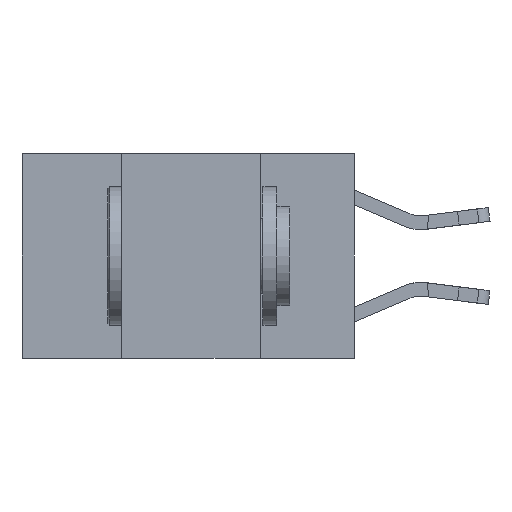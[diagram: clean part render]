
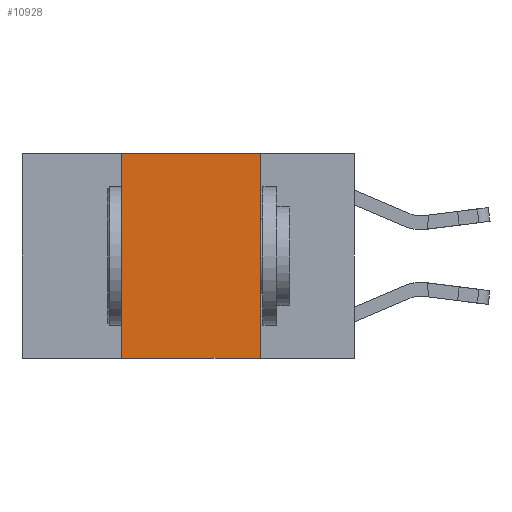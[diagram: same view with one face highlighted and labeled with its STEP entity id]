
A CAD part, left-side view. The second image highlights one B-rep face of the part: STEP entity #10928.
In plain terms, the highlighted planar face has unit normal (-1, 0, 0).
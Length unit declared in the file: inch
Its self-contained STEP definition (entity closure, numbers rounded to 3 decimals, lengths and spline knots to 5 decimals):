
#56 = VERTEX_POINT ( 'NONE', #12856 ) ;
#953 = CARTESIAN_POINT ( 'NONE',  ( 0., 0.6, -0.37 ) ) ;
#1276 = PLANE ( 'NONE',  #14299 ) ;
#2473 = DIRECTION ( 'NONE',  ( 0., -1., 0. ) ) ;
#2600 = DIRECTION ( 'NONE',  ( 1., 0., 0. ) ) ;
#2632 = ORIENTED_EDGE ( 'NONE', *, *, #9256, .F. ) ;
#3325 = LINE ( 'NONE', #12449, #12921 ) ;
#3659 = CARTESIAN_POINT ( 'NONE',  ( 0., 0.42, 0. ) ) ;
#4033 = ORIENTED_EDGE ( 'NONE', *, *, #9670, .F. ) ;
#4121 = ORIENTED_EDGE ( 'NONE', *, *, #9251, .F. ) ;
#5117 = ORIENTED_EDGE ( 'NONE', *, *, #9229, .T. ) ;
#6235 = DIRECTION ( 'NONE',  ( 0., -1., 0. ) ) ;
#6783 = VECTOR ( 'NONE', #6235, 39.37008 ) ;
#7540 = DIRECTION ( 'NONE',  ( 0., 0., -1. ) ) ;
#7731 = CARTESIAN_POINT ( 'NONE',  ( 0., 0.6, 0. ) ) ;
#7838 = VERTEX_POINT ( 'NONE', #14112 ) ;
#9226 = CARTESIAN_POINT ( 'NONE',  ( 0., 0.17, -0.37 ) ) ;
#9229 = EDGE_CURVE ( 'NONE', #7838, #14200, #10879, .T. ) ;
#9251 = EDGE_CURVE ( 'NONE', #7838, #10206, #10136, .T. ) ;
#9256 = EDGE_CURVE ( 'NONE', #56, #14200, #3325, .T. ) ;
#9670 = EDGE_CURVE ( 'NONE', #10206, #56, #14014, .T. ) ;
#9770 = VECTOR ( 'NONE', #13605, 39.37008 ) ;
#10136 = LINE ( 'NONE', #3659, #9770 ) ;
#10206 = VERTEX_POINT ( 'NONE', #11046 ) ;
#10664 = EDGE_LOOP ( 'NONE', ( #2632, #4033, #4121, #5117 ) ) ;
#10879 = LINE ( 'NONE', #953, #6783 ) ;
#10882 = VECTOR ( 'NONE', #2473, 39.37008 ) ;
#10928 = ADVANCED_FACE ( 'NONE', ( #15238 ), #1276, .F. ) ;
#11046 = CARTESIAN_POINT ( 'NONE',  ( 0., 0.42, 0. ) ) ;
#11366 = CARTESIAN_POINT ( 'NONE',  ( 0., 0.6, 0. ) ) ;
#11470 = DIRECTION ( 'NONE',  ( 0., 0., -1. ) ) ;
#12449 = CARTESIAN_POINT ( 'NONE',  ( 0., 0.17, 0. ) ) ;
#12856 = CARTESIAN_POINT ( 'NONE',  ( 0., 0.17, 0. ) ) ;
#12921 = VECTOR ( 'NONE', #7540, 39.37008 ) ;
#13605 = DIRECTION ( 'NONE',  ( 0., 0., 1. ) ) ;
#14014 = LINE ( 'NONE', #11366, #10882 ) ;
#14112 = CARTESIAN_POINT ( 'NONE',  ( 0., 0.42, -0.37 ) ) ;
#14200 = VERTEX_POINT ( 'NONE', #9226 ) ;
#14299 = AXIS2_PLACEMENT_3D ( 'NONE', #7731, #2600, #11470 ) ;
#15238 = FACE_OUTER_BOUND ( 'NONE', #10664, .T. ) ;
